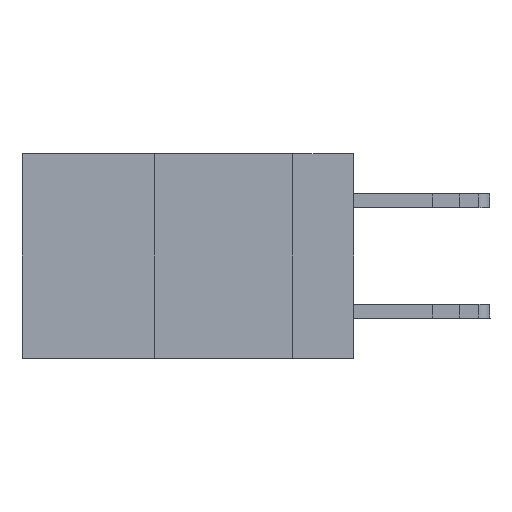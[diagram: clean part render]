
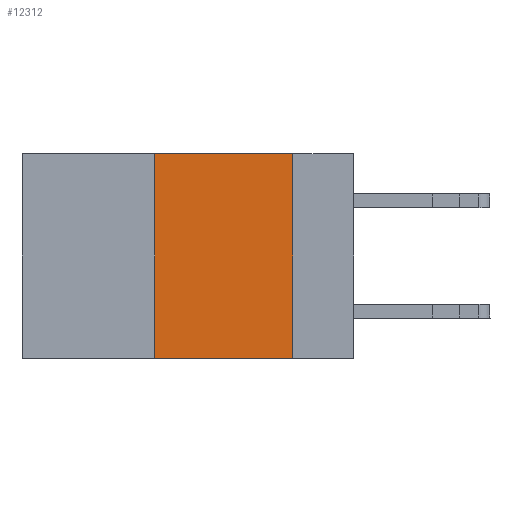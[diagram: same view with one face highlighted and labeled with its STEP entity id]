
A CAD part, left-side view. The second image highlights one B-rep face of the part: STEP entity #12312.
In plain terms, the highlighted planar face has unit normal (-1, 0, 0).
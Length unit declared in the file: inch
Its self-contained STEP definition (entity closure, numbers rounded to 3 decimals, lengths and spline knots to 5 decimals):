
#267 = EDGE_LOOP ( 'NONE', ( #26204, #22087, #8908, #31762 ) ) ;
#1218 = AXIS2_PLACEMENT_3D ( 'NONE', #18424, #31481, #18768 ) ;
#1963 = LINE ( 'NONE', #20919, #28666 ) ;
#3884 = CARTESIAN_POINT ( 'NONE',  ( 0., 0.6, -0.37 ) ) ;
#4421 = CARTESIAN_POINT ( 'NONE',  ( 0., 0.11, 0. ) ) ;
#6896 = VERTEX_POINT ( 'NONE', #12336 ) ;
#7880 = CARTESIAN_POINT ( 'NONE',  ( 0., 0.11, 0. ) ) ;
#8163 = FACE_OUTER_BOUND ( 'NONE', #267, .T. ) ;
#8435 = PLANE ( 'NONE',  #1218 ) ;
#8908 = ORIENTED_EDGE ( 'NONE', *, *, #16583, .F. ) ;
#11792 = CARTESIAN_POINT ( 'NONE',  ( 0., 0.11, -0.37 ) ) ;
#12092 = DIRECTION ( 'NONE',  ( 0., 0., -1. ) ) ;
#12312 = ADVANCED_FACE ( 'NONE', ( #8163 ), #8435, .F. ) ;
#12336 = CARTESIAN_POINT ( 'NONE',  ( 0., 0.36, -0.37 ) ) ;
#13444 = CARTESIAN_POINT ( 'NONE',  ( 0., 0.36, 0. ) ) ;
#15624 = VERTEX_POINT ( 'NONE', #22970 ) ;
#16054 = VECTOR ( 'NONE', #12092, 39.37008 ) ;
#16187 = DIRECTION ( 'NONE',  ( 0., -1., 0. ) ) ;
#16583 = EDGE_CURVE ( 'NONE', #6896, #15624, #28564, .T. ) ;
#18424 = CARTESIAN_POINT ( 'NONE',  ( 0., 0.6, 0. ) ) ;
#18768 = DIRECTION ( 'NONE',  ( 0., 0., -1. ) ) ;
#20919 = CARTESIAN_POINT ( 'NONE',  ( 0., 0.6, 0. ) ) ;
#21245 = LINE ( 'NONE', #4421, #16054 ) ;
#21277 = EDGE_CURVE ( 'NONE', #6896, #23017, #28506, .T. ) ;
#21720 = DIRECTION ( 'NONE',  ( 0., -1., 0. ) ) ;
#21742 = VECTOR ( 'NONE', #21720, 39.37008 ) ;
#22087 = ORIENTED_EDGE ( 'NONE', *, *, #32636, .F. ) ;
#22970 = CARTESIAN_POINT ( 'NONE',  ( 0., 0.36, 0. ) ) ;
#23017 = VERTEX_POINT ( 'NONE', #11792 ) ;
#25486 = DIRECTION ( 'NONE',  ( 0., 0., 1. ) ) ;
#26204 = ORIENTED_EDGE ( 'NONE', *, *, #26984, .F. ) ;
#26984 = EDGE_CURVE ( 'NONE', #31610, #23017, #21245, .T. ) ;
#28506 = LINE ( 'NONE', #3884, #21742 ) ;
#28564 = LINE ( 'NONE', #13444, #32944 ) ;
#28666 = VECTOR ( 'NONE', #16187, 39.37008 ) ;
#31481 = DIRECTION ( 'NONE',  ( 1., 0., 0. ) ) ;
#31610 = VERTEX_POINT ( 'NONE', #7880 ) ;
#31762 = ORIENTED_EDGE ( 'NONE', *, *, #21277, .T. ) ;
#32636 = EDGE_CURVE ( 'NONE', #15624, #31610, #1963, .T. ) ;
#32944 = VECTOR ( 'NONE', #25486, 39.37008 ) ;
